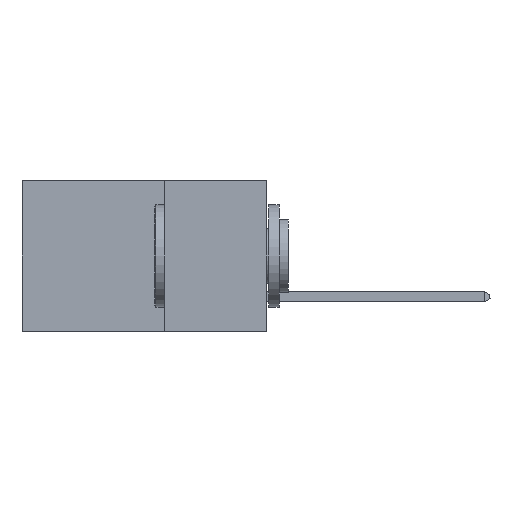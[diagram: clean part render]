
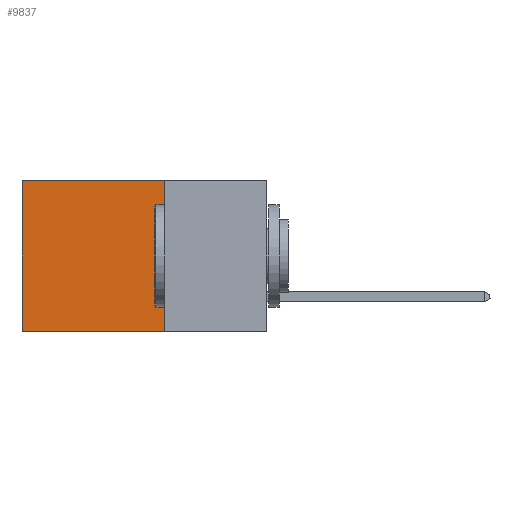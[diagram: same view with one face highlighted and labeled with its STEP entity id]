
A CAD part, left-side view. The second image highlights one B-rep face of the part: STEP entity #9837.
In plain terms, the highlighted planar face has unit normal (-1, 0, 0).
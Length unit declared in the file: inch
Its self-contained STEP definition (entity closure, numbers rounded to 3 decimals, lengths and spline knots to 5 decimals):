
#2859 = DIRECTION ( 'NONE',  ( 0., 1., 0. ) ) ;
#5366 = DIRECTION ( 'NONE',  ( 1., 0., 0. ) ) ;
#5592 = CARTESIAN_POINT ( 'NONE',  ( 0.2875, 0.6, 0. ) ) ;
#5819 = ORIENTED_EDGE ( 'NONE', *, *, #20004, .T. ) ;
#6692 = ORIENTED_EDGE ( 'NONE', *, *, #10380, .F. ) ;
#7402 = CARTESIAN_POINT ( 'NONE',  ( 0.2875, 0.25, -0.37 ) ) ;
#7784 = VECTOR ( 'NONE', #9386, 39.37008 ) ;
#7944 = VECTOR ( 'NONE', #21212, 39.37008 ) ;
#8084 = AXIS2_PLACEMENT_3D ( 'NONE', #16143, #5366, #16475 ) ;
#8445 = EDGE_CURVE ( 'NONE', #18810, #10023, #12736, .T. ) ;
#8941 = VERTEX_POINT ( 'NONE', #23278 ) ;
#9386 = DIRECTION ( 'NONE',  ( 0., 0., -1. ) ) ;
#9837 = ADVANCED_FACE ( 'NONE', ( #15831 ), #11072, .F. ) ;
#10023 = VERTEX_POINT ( 'NONE', #7402 ) ;
#10380 = EDGE_CURVE ( 'NONE', #10023, #8941, #11526, .T. ) ;
#10456 = CARTESIAN_POINT ( 'NONE',  ( 0.2875, 0.25, 0. ) ) ;
#10893 = LINE ( 'NONE', #10456, #16308 ) ;
#11072 = PLANE ( 'NONE',  #8084 ) ;
#11345 = EDGE_CURVE ( 'NONE', #17771, #8941, #23415, .T. ) ;
#11526 = LINE ( 'NONE', #13817, #21226 ) ;
#12736 = LINE ( 'NONE', #17570, #7944 ) ;
#13817 = CARTESIAN_POINT ( 'NONE',  ( 0.2875, 0.25, -0.37 ) ) ;
#15831 = FACE_OUTER_BOUND ( 'NONE', #22751, .T. ) ;
#15842 = ORIENTED_EDGE ( 'NONE', *, *, #8445, .F. ) ;
#16143 = CARTESIAN_POINT ( 'NONE',  ( 0.2875, 0.25, 0. ) ) ;
#16268 = ORIENTED_EDGE ( 'NONE', *, *, #11345, .T. ) ;
#16308 = VECTOR ( 'NONE', #21090, 39.37008 ) ;
#16475 = DIRECTION ( 'NONE',  ( 0., 0., -1. ) ) ;
#17570 = CARTESIAN_POINT ( 'NONE',  ( 0.2875, 0.25, 0. ) ) ;
#17771 = VERTEX_POINT ( 'NONE', #5592 ) ;
#18259 = CARTESIAN_POINT ( 'NONE',  ( 0.2875, 0.25, 0. ) ) ;
#18810 = VERTEX_POINT ( 'NONE', #18259 ) ;
#19662 = CARTESIAN_POINT ( 'NONE',  ( 0.2875, 0.6, 0. ) ) ;
#20004 = EDGE_CURVE ( 'NONE', #18810, #17771, #10893, .T. ) ;
#21090 = DIRECTION ( 'NONE',  ( 0., 1., 0. ) ) ;
#21212 = DIRECTION ( 'NONE',  ( 0., 0., -1. ) ) ;
#21226 = VECTOR ( 'NONE', #2859, 39.37008 ) ;
#22751 = EDGE_LOOP ( 'NONE', ( #16268, #6692, #15842, #5819 ) ) ;
#23278 = CARTESIAN_POINT ( 'NONE',  ( 0.2875, 0.6, -0.37 ) ) ;
#23415 = LINE ( 'NONE', #19662, #7784 ) ;
